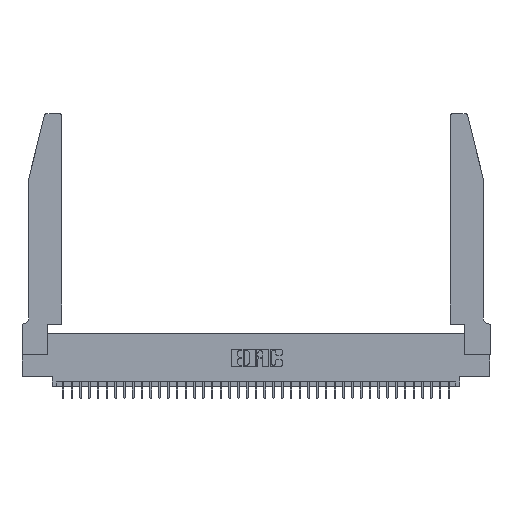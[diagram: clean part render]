
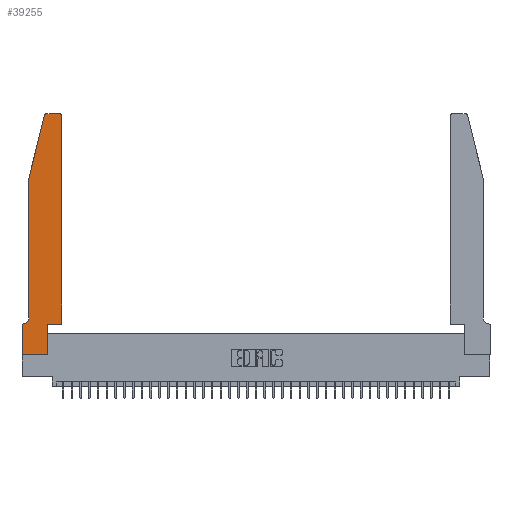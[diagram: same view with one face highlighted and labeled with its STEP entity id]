
A CAD part, top view. The second image highlights one B-rep face of the part: STEP entity #39255.
In plain terms, the highlighted planar face has unit normal (0, 0, 1).
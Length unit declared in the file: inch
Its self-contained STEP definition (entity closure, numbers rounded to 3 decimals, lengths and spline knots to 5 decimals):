
#53 = DIRECTION ( 'NONE',  ( 0., 0., 1. ) ) ;
#705 = CARTESIAN_POINT ( 'NONE',  ( 0., 0., 0.37 ) ) ;
#838 = VERTEX_POINT ( 'NONE', #39104 ) ;
#845 = CARTESIAN_POINT ( 'NONE',  ( 0.0755, 2., 0.37 ) ) ;
#1236 = VERTEX_POINT ( 'NONE', #4327 ) ;
#1362 = AXIS2_PLACEMENT_3D ( 'NONE', #11482, #8452, #39161 ) ;
#2267 = CARTESIAN_POINT ( 'NONE',  ( 0., 0.35, 0.37 ) ) ;
#2290 = DIRECTION ( 'NONE',  ( 0., 0., 1. ) ) ;
#2427 = CARTESIAN_POINT ( 'NONE',  ( 0.2605, 2.75, 0.37 ) ) ;
#2558 = CARTESIAN_POINT ( 'NONE',  ( 0., 0., 0.37 ) ) ;
#2644 = VERTEX_POINT ( 'NONE', #8744 ) ;
#3914 = LINE ( 'NONE', #37829, #33420 ) ;
#4327 = CARTESIAN_POINT ( 'NONE',  ( 0.4505, 0.35, 0.37 ) ) ;
#4393 = EDGE_CURVE ( 'NONE', #9509, #31392, #3914, .T. ) ;
#4560 = ORIENTED_EDGE ( 'NONE', *, *, #18114, .T. ) ;
#4938 = CARTESIAN_POINT ( 'NONE',  ( 0.284, 2.72, 0.37 ) ) ;
#5265 = CARTESIAN_POINT ( 'NONE',  ( 0.0055, 0.35, 0.37 ) ) ;
#6804 = EDGE_CURVE ( 'NONE', #20823, #22931, #31495, .T. ) ;
#6947 = LINE ( 'NONE', #705, #25423 ) ;
#7172 = EDGE_CURVE ( 'NONE', #31392, #16918, #10716, .T. ) ;
#7692 = VERTEX_POINT ( 'NONE', #37845 ) ;
#8452 = DIRECTION ( 'NONE',  ( 0., 0., 1. ) ) ;
#8744 = CARTESIAN_POINT ( 'NONE',  ( 0.2865, 0.35, 0.37 ) ) ;
#9509 = VERTEX_POINT ( 'NONE', #31588 ) ;
#9714 = EDGE_LOOP ( 'NONE', ( #17029, #35402, #25635, #22762, #31978, #31267, #25754, #20155, #4560, #19218, #20227, #23570 ) ) ;
#9836 = DIRECTION ( 'NONE',  ( -1., 0., 0. ) ) ;
#10170 = CARTESIAN_POINT ( 'NONE',  ( 0.2865, 0.35, 0.37 ) ) ;
#10683 = AXIS2_PLACEMENT_3D ( 'NONE', #4938, #2290, #27149 ) ;
#10716 = CIRCLE ( 'NONE', #38451, 0.07 ) ;
#10734 = CIRCLE ( 'NONE', #37836, 0.03 ) ;
#11482 = CARTESIAN_POINT ( 'NONE',  ( 0., 0.35, 0.37 ) ) ;
#11767 = CARTESIAN_POINT ( 'NONE',  ( 0.2865, 0., 0.37 ) ) ;
#11966 = CARTESIAN_POINT ( 'NONE',  ( 0.4205, 2.72, 0.37 ) ) ;
#12472 = CARTESIAN_POINT ( 'NONE',  ( 0.0755, 0.35, 0.37 ) ) ;
#12552 = VECTOR ( 'NONE', #9836, 39.37008 ) ;
#12909 = CARTESIAN_POINT ( 'NONE',  ( 0., 0., 0.37 ) ) ;
#13026 = DIRECTION ( 'NONE',  ( 0., -1., 0. ) ) ;
#13167 = VECTOR ( 'NONE', #31408, 39.37008 ) ;
#13171 = DIRECTION ( 'NONE',  ( -0.239, -0.971, 0. ) ) ;
#13794 = DIRECTION ( 'NONE',  ( 0., -1., 0. ) ) ;
#14125 = CARTESIAN_POINT ( 'NONE',  ( 0.0755, 0.42, 0.37 ) ) ;
#15191 = DIRECTION ( 'NONE',  ( 1., 0., 0. ) ) ;
#15599 = VERTEX_POINT ( 'NONE', #31398 ) ;
#15918 = DIRECTION ( 'NONE',  ( 0., 0., -1. ) ) ;
#16132 = DIRECTION ( 'NONE',  ( 0., 1., 0. ) ) ;
#16918 = VERTEX_POINT ( 'NONE', #5265 ) ;
#17029 = ORIENTED_EDGE ( 'NONE', *, *, #37483, .T. ) ;
#18114 = EDGE_CURVE ( 'NONE', #22931, #2644, #35210, .T. ) ;
#18700 = CIRCLE ( 'NONE', #10683, 0.03 ) ;
#18774 = EDGE_CURVE ( 'NONE', #16918, #26400, #31465, .T. ) ;
#19153 = LINE ( 'NONE', #31475, #23345 ) ;
#19218 = ORIENTED_EDGE ( 'NONE', *, *, #32200, .T. ) ;
#20155 = ORIENTED_EDGE ( 'NONE', *, *, #6804, .T. ) ;
#20227 = ORIENTED_EDGE ( 'NONE', *, *, #39673, .T. ) ;
#20823 = VERTEX_POINT ( 'NONE', #2558 ) ;
#21466 = DIRECTION ( 'NONE',  ( 1., 0., 0. ) ) ;
#22547 = CARTESIAN_POINT ( 'NONE',  ( 0.0055, 0.42, 0.37 ) ) ;
#22548 = VECTOR ( 'NONE', #23268, 39.37008 ) ;
#22762 = ORIENTED_EDGE ( 'NONE', *, *, #4393, .T. ) ;
#22881 = EDGE_CURVE ( 'NONE', #7692, #30068, #10734, .T. ) ;
#22931 = VERTEX_POINT ( 'NONE', #11767 ) ;
#23268 = DIRECTION ( 'NONE',  ( -1., 0., 0. ) ) ;
#23345 = VECTOR ( 'NONE', #16132, 39.37008 ) ;
#23570 = ORIENTED_EDGE ( 'NONE', *, *, #22881, .T. ) ;
#24365 = EDGE_CURVE ( 'NONE', #838, #9509, #31547, .T. ) ;
#24972 = CARTESIAN_POINT ( 'NONE',  ( 0.4205, 2.75, 0.37 ) ) ;
#25423 = VECTOR ( 'NONE', #13026, 39.37008 ) ;
#25635 = ORIENTED_EDGE ( 'NONE', *, *, #24365, .T. ) ;
#25754 = ORIENTED_EDGE ( 'NONE', *, *, #33796, .T. ) ;
#26400 = VERTEX_POINT ( 'NONE', #2267 ) ;
#26901 = LINE ( 'NONE', #2427, #22548 ) ;
#27149 = DIRECTION ( 'NONE',  ( 1., 0., 0. ) ) ;
#28126 = VECTOR ( 'NONE', #34709, 39.37008 ) ;
#30068 = VERTEX_POINT ( 'NONE', #24972 ) ;
#30186 = VECTOR ( 'NONE', #13171, 39.37008 ) ;
#31267 = ORIENTED_EDGE ( 'NONE', *, *, #18774, .T. ) ;
#31392 = VERTEX_POINT ( 'NONE', #14125 ) ;
#31398 = CARTESIAN_POINT ( 'NONE',  ( 0.284, 2.75, 0.37 ) ) ;
#31408 = DIRECTION ( 'NONE',  ( 0., 1., 0. ) ) ;
#31465 = LINE ( 'NONE', #12472, #12552 ) ;
#31475 = CARTESIAN_POINT ( 'NONE',  ( 0.4505, 0.35, 0.37 ) ) ;
#31495 = LINE ( 'NONE', #12909, #28126 ) ;
#31547 = LINE ( 'NONE', #845, #30186 ) ;
#31588 = CARTESIAN_POINT ( 'NONE',  ( 0.0755, 2., 0.37 ) ) ;
#31978 = ORIENTED_EDGE ( 'NONE', *, *, #7172, .T. ) ;
#32200 = EDGE_CURVE ( 'NONE', #2644, #1236, #33173, .T. ) ;
#32708 = PLANE ( 'NONE',  #1362 ) ;
#33173 = LINE ( 'NONE', #39423, #36930 ) ;
#33420 = VECTOR ( 'NONE', #13794, 39.37008 ) ;
#33796 = EDGE_CURVE ( 'NONE', #26400, #20823, #6947, .T. ) ;
#34709 = DIRECTION ( 'NONE',  ( 1., 0., 0. ) ) ;
#34863 = DIRECTION ( 'NONE',  ( -1., 0., 0. ) ) ;
#35210 = LINE ( 'NONE', #10170, #13167 ) ;
#35402 = ORIENTED_EDGE ( 'NONE', *, *, #37216, .T. ) ;
#35926 = FACE_OUTER_BOUND ( 'NONE', #9714, .T. ) ;
#36930 = VECTOR ( 'NONE', #15191, 39.37008 ) ;
#37216 = EDGE_CURVE ( 'NONE', #15599, #838, #18700, .T. ) ;
#37483 = EDGE_CURVE ( 'NONE', #30068, #15599, #26901, .T. ) ;
#37829 = CARTESIAN_POINT ( 'NONE',  ( 0.0755, 2., 0.37 ) ) ;
#37836 = AXIS2_PLACEMENT_3D ( 'NONE', #11966, #53, #21466 ) ;
#37845 = CARTESIAN_POINT ( 'NONE',  ( 0.4505, 2.72, 0.37 ) ) ;
#38451 = AXIS2_PLACEMENT_3D ( 'NONE', #22547, #15918, #34863 ) ;
#39104 = CARTESIAN_POINT ( 'NONE',  ( 0.25487, 2.72718, 0.37 ) ) ;
#39161 = DIRECTION ( 'NONE',  ( 1., 0., 0. ) ) ;
#39255 = ADVANCED_FACE ( 'NONE', ( #35926 ), #32708, .T. ) ;
#39423 = CARTESIAN_POINT ( 'NONE',  ( 0.4505, 0.35, 0.37 ) ) ;
#39673 = EDGE_CURVE ( 'NONE', #1236, #7692, #19153, .T. ) ;
